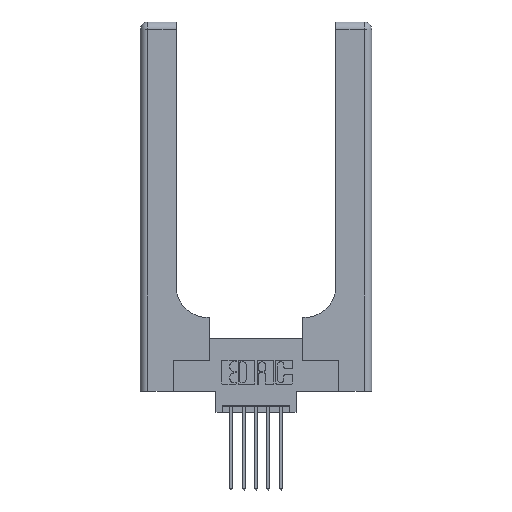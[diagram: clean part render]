
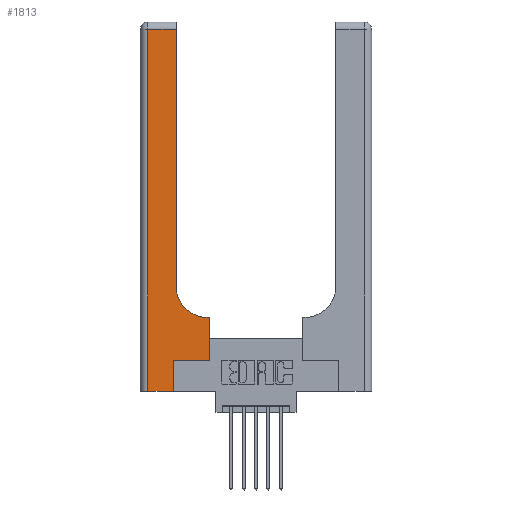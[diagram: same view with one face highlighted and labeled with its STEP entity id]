
A CAD part, top view. The second image highlights one B-rep face of the part: STEP entity #1813.
In plain terms, the highlighted planar face has unit normal (0, 0, 1).
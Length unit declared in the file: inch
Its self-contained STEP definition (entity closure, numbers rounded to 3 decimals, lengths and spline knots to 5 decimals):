
#220 = CARTESIAN_POINT ( 'NONE',  ( 0., 2.94, 0.37 ) ) ;
#384 = ORIENTED_EDGE ( 'NONE', *, *, #6422, .T. ) ;
#393 = CARTESIAN_POINT ( 'NONE',  ( 0.2915, 2.94, 0.37 ) ) ;
#498 = CARTESIAN_POINT ( 'NONE',  ( 0., 0., 0.37 ) ) ;
#913 = CARTESIAN_POINT ( 'NONE',  ( 0.5585, 0.25, 0.37 ) ) ;
#1409 = CARTESIAN_POINT ( 'NONE',  ( 0.5415, 0.6, 0.37 ) ) ;
#1493 = LINE ( 'NONE', #10851, #10210 ) ;
#1585 = DIRECTION ( 'NONE',  ( 1., 0., 0. ) ) ;
#1813 = ADVANCED_FACE ( 'NONE', ( #1856 ), #2951, .F. ) ;
#1829 = VERTEX_POINT ( 'NONE', #2965 ) ;
#1856 = FACE_OUTER_BOUND ( 'NONE', #11460, .T. ) ;
#1953 = VECTOR ( 'NONE', #1585, 39.37008 ) ;
#2014 = LINE ( 'NONE', #13337, #10722 ) ;
#2323 = LINE ( 'NONE', #498, #1953 ) ;
#2409 = CARTESIAN_POINT ( 'NONE',  ( 0.06, 0., 0.37 ) ) ;
#2827 = CARTESIAN_POINT ( 'NONE',  ( 0.269, 0.25, 0.37 ) ) ;
#2909 = DIRECTION ( 'NONE',  ( -1., 0., 0. ) ) ;
#2913 = EDGE_CURVE ( 'NONE', #4453, #8752, #9865, .T. ) ;
#2914 = DIRECTION ( 'NONE',  ( 0., 0., -1. ) ) ;
#2951 = PLANE ( 'NONE',  #9264 ) ;
#2965 = CARTESIAN_POINT ( 'NONE',  ( 0.5585, 0.6, 0.37 ) ) ;
#3077 = CARTESIAN_POINT ( 'NONE',  ( 0., 3., 0.37 ) ) ;
#3258 = DIRECTION ( 'NONE',  ( 0., 1., 0. ) ) ;
#4159 = ORIENTED_EDGE ( 'NONE', *, *, #9912, .T. ) ;
#4453 = VERTEX_POINT ( 'NONE', #2827 ) ;
#4674 = VERTEX_POINT ( 'NONE', #2409 ) ;
#4840 = CARTESIAN_POINT ( 'NONE',  ( 0.269, 0., 0.37 ) ) ;
#4956 = CARTESIAN_POINT ( 'NONE',  ( 0.5415, 0.85, 0.37 ) ) ;
#5500 = EDGE_CURVE ( 'NONE', #7525, #8345, #11374, .T. ) ;
#5542 = EDGE_CURVE ( 'NONE', #4674, #13997, #2323, .T. ) ;
#6073 = DIRECTION ( 'NONE',  ( 1., 0., 0. ) ) ;
#6422 = EDGE_CURVE ( 'NONE', #11693, #7273, #6661, .T. ) ;
#6431 = DIRECTION ( 'NONE',  ( 1., 0., 0. ) ) ;
#6434 = CARTESIAN_POINT ( 'NONE',  ( 0.269, 0.25, 0.37 ) ) ;
#6451 = VECTOR ( 'NONE', #8050, 39.37008 ) ;
#6571 = DIRECTION ( 'NONE',  ( 0., -1., 0. ) ) ;
#6661 = LINE ( 'NONE', #220, #12047 ) ;
#6892 = DIRECTION ( 'NONE',  ( -1., 0., 0. ) ) ;
#6934 = CARTESIAN_POINT ( 'NONE',  ( 0.2915, 3., 0.37 ) ) ;
#7084 = VECTOR ( 'NONE', #6431, 39.37008 ) ;
#7092 = ORIENTED_EDGE ( 'NONE', *, *, #2913, .T. ) ;
#7273 = VERTEX_POINT ( 'NONE', #10797 ) ;
#7525 = VERTEX_POINT ( 'NONE', #1409 ) ;
#7747 = ORIENTED_EDGE ( 'NONE', *, *, #5500, .T. ) ;
#8050 = DIRECTION ( 'NONE',  ( 0., 1., 0. ) ) ;
#8345 = VERTEX_POINT ( 'NONE', #11989 ) ;
#8752 = VERTEX_POINT ( 'NONE', #12632 ) ;
#9098 = DIRECTION ( 'NONE',  ( -1., 0., 0. ) ) ;
#9215 = ORIENTED_EDGE ( 'NONE', *, *, #10227, .T. ) ;
#9254 = LINE ( 'NONE', #6934, #6451 ) ;
#9264 = AXIS2_PLACEMENT_3D ( 'NONE', #3077, #2914, #2909 ) ;
#9865 = LINE ( 'NONE', #6434, #7084 ) ;
#9868 = VECTOR ( 'NONE', #3258, 39.37008 ) ;
#9912 = EDGE_CURVE ( 'NONE', #13997, #4453, #11101, .T. ) ;
#10210 = VECTOR ( 'NONE', #6571, 39.37008 ) ;
#10214 = ORIENTED_EDGE ( 'NONE', *, *, #10219, .T. ) ;
#10219 = EDGE_CURVE ( 'NONE', #8752, #1829, #12808, .T. ) ;
#10227 = EDGE_CURVE ( 'NONE', #7273, #4674, #1493, .T. ) ;
#10394 = EDGE_CURVE ( 'NONE', #1829, #7525, #2014, .T. ) ;
#10722 = VECTOR ( 'NONE', #6892, 39.37008 ) ;
#10797 = CARTESIAN_POINT ( 'NONE',  ( 0.06, 2.94, 0.37 ) ) ;
#10851 = CARTESIAN_POINT ( 'NONE',  ( 0.06, 3., 0.37 ) ) ;
#11101 = LINE ( 'NONE', #4840, #13965 ) ;
#11306 = DIRECTION ( 'NONE',  ( 0., 1., 0. ) ) ;
#11374 = CIRCLE ( 'NONE', #13905, 0.25 ) ;
#11460 = EDGE_LOOP ( 'NONE', ( #11787, #384, #9215, #12123, #4159, #7092, #10214, #13150, #7747 ) ) ;
#11693 = VERTEX_POINT ( 'NONE', #393 ) ;
#11787 = ORIENTED_EDGE ( 'NONE', *, *, #12251, .T. ) ;
#11989 = CARTESIAN_POINT ( 'NONE',  ( 0.2915, 0.85, 0.37 ) ) ;
#12047 = VECTOR ( 'NONE', #9098, 39.37008 ) ;
#12123 = ORIENTED_EDGE ( 'NONE', *, *, #5542, .T. ) ;
#12251 = EDGE_CURVE ( 'NONE', #8345, #11693, #9254, .T. ) ;
#12473 = CARTESIAN_POINT ( 'NONE',  ( 0.269, 0., 0.37 ) ) ;
#12507 = DIRECTION ( 'NONE',  ( 0., 0., -1. ) ) ;
#12632 = CARTESIAN_POINT ( 'NONE',  ( 0.5585, 0.25, 0.37 ) ) ;
#12808 = LINE ( 'NONE', #913, #9868 ) ;
#13150 = ORIENTED_EDGE ( 'NONE', *, *, #10394, .T. ) ;
#13337 = CARTESIAN_POINT ( 'NONE',  ( 0.2915, 0.6, 0.37 ) ) ;
#13905 = AXIS2_PLACEMENT_3D ( 'NONE', #4956, #12507, #6073 ) ;
#13965 = VECTOR ( 'NONE', #11306, 39.37008 ) ;
#13997 = VERTEX_POINT ( 'NONE', #12473 ) ;
